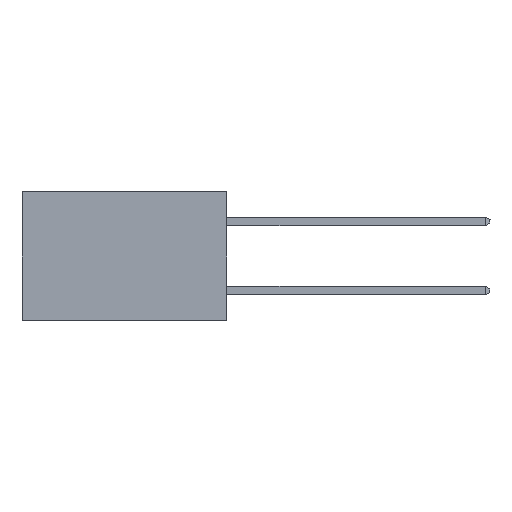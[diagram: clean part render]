
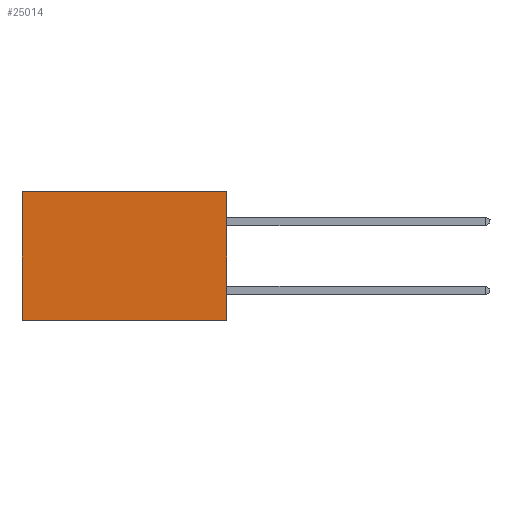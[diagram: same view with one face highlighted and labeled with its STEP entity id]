
A CAD part, left-side view. The second image highlights one B-rep face of the part: STEP entity #25014.
In plain terms, the highlighted planar face has unit normal (-1, 0, 0).
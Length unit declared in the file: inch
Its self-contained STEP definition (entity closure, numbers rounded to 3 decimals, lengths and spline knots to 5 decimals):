
#579 = VECTOR ( 'NONE', #823, 39.37008 ) ;
#823 = DIRECTION ( 'NONE',  ( 0., 0., -1. ) ) ;
#1148 = VERTEX_POINT ( 'NONE', #10219 ) ;
#1304 = ORIENTED_EDGE ( 'NONE', *, *, #18436, .T. ) ;
#1668 = VERTEX_POINT ( 'NONE', #4537 ) ;
#2913 = VERTEX_POINT ( 'NONE', #23865 ) ;
#3232 = DIRECTION ( 'NONE',  ( 1., 0., 0. ) ) ;
#4537 = CARTESIAN_POINT ( 'NONE',  ( 0.277, 0., 0. ) ) ;
#4989 = EDGE_CURVE ( 'NONE', #30643, #1148, #21159, .T. ) ;
#5050 = FACE_OUTER_BOUND ( 'NONE', #31532, .T. ) ;
#5463 = ORIENTED_EDGE ( 'NONE', *, *, #33277, .F. ) ;
#5634 = DIRECTION ( 'NONE',  ( 0., 1., 0. ) ) ;
#5979 = LINE ( 'NONE', #16574, #579 ) ;
#7530 = CARTESIAN_POINT ( 'NONE',  ( 0.277, 0., -0.37 ) ) ;
#7658 = LINE ( 'NONE', #18670, #20694 ) ;
#10193 = DIRECTION ( 'NONE',  ( 0., 1., 0. ) ) ;
#10219 = CARTESIAN_POINT ( 'NONE',  ( 0.277, 0.59, -0.37 ) ) ;
#11895 = CARTESIAN_POINT ( 'NONE',  ( 0.277, 0.59, 0. ) ) ;
#12642 = ORIENTED_EDGE ( 'NONE', *, *, #4989, .T. ) ;
#12999 = EDGE_CURVE ( 'NONE', #2913, #1148, #29421, .T. ) ;
#13694 = CARTESIAN_POINT ( 'NONE',  ( 0.277, 0., -0.37 ) ) ;
#14587 = ORIENTED_EDGE ( 'NONE', *, *, #12999, .F. ) ;
#14934 = VECTOR ( 'NONE', #10193, 39.37008 ) ;
#16574 = CARTESIAN_POINT ( 'NONE',  ( 0.277, 0., -0.37 ) ) ;
#16748 = DIRECTION ( 'NONE',  ( 0., 0., -1. ) ) ;
#18336 = CARTESIAN_POINT ( 'NONE',  ( 0.277, 0.59, -0.37 ) ) ;
#18436 = EDGE_CURVE ( 'NONE', #1668, #30643, #7658, .T. ) ;
#18670 = CARTESIAN_POINT ( 'NONE',  ( 0.277, 0., 0. ) ) ;
#20694 = VECTOR ( 'NONE', #5634, 39.37008 ) ;
#21159 = LINE ( 'NONE', #18336, #27155 ) ;
#21372 = PLANE ( 'NONE',  #29951 ) ;
#21485 = DIRECTION ( 'NONE',  ( 0., 0., -1. ) ) ;
#23865 = CARTESIAN_POINT ( 'NONE',  ( 0.277, 0., -0.37 ) ) ;
#25014 = ADVANCED_FACE ( 'NONE', ( #5050 ), #21372, .F. ) ;
#27155 = VECTOR ( 'NONE', #16748, 39.37008 ) ;
#29421 = LINE ( 'NONE', #7530, #14934 ) ;
#29951 = AXIS2_PLACEMENT_3D ( 'NONE', #13694, #3232, #21485 ) ;
#30643 = VERTEX_POINT ( 'NONE', #11895 ) ;
#31532 = EDGE_LOOP ( 'NONE', ( #12642, #14587, #5463, #1304 ) ) ;
#33277 = EDGE_CURVE ( 'NONE', #1668, #2913, #5979, .T. ) ;
